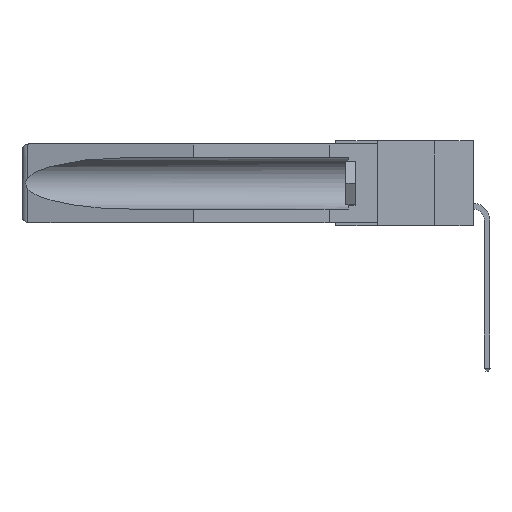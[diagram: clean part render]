
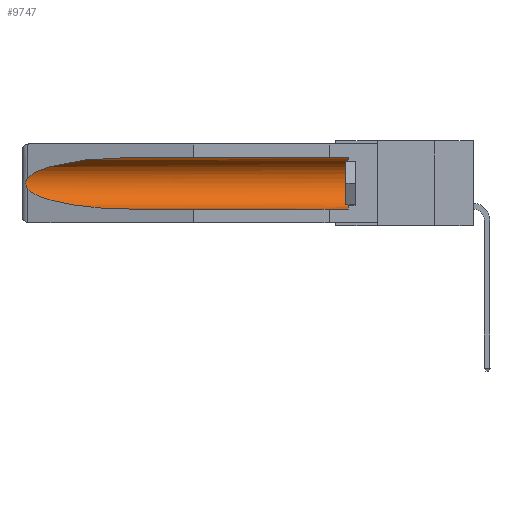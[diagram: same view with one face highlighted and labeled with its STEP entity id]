
A CAD part, left-side view. The second image highlights one B-rep face of the part: STEP entity #9747.
In plain terms, the highlighted cylindrical face has radius 2.857 mm (diameter 5.715 mm), a partial arc.
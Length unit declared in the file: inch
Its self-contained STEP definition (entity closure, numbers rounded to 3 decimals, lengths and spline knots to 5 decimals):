
#97 = CARTESIAN_POINT ( 'NONE',  ( 0.21114, 1.30732, -0.284 ) ) ;
#556 = CARTESIAN_POINT ( 'NONE',  ( 0.26537, 1.52718, -0.14972 ) ) ;
#1008 = DIRECTION ( 'NONE',  ( 0., -1., 0. ) ) ;
#1019 = CARTESIAN_POINT ( 'NONE',  ( 0.155, 0.126, -0.059 ) ) ;
#2188 = CARTESIAN_POINT ( 'NONE',  ( 0.155, 0.126, -0.284 ) ) ;
#2628 = CARTESIAN_POINT ( 'NONE',  ( 0.2673, 1.53269, -0.17917 ) ) ;
#2729 = CARTESIAN_POINT ( 'NONE',  ( 0.26537, 1.52718, -0.19328 ) ) ;
#3008 = FACE_OUTER_BOUND ( 'NONE', #10866, .T. ) ;
#3377 =( BOUNDED_CURVE ( )  B_SPLINE_CURVE ( 3, ( #17045, #12734, #97, #4221 ),
 .UNSPECIFIED., .F., .F. ) 
 B_SPLINE_CURVE_WITH_KNOTS ( ( 4, 4 ),
 ( 0.1948, 1.5708 ),
 .UNSPECIFIED. ) 
 CURVE ( )  GEOMETRIC_REPRESENTATION_ITEM ( )  RATIONAL_B_SPLINE_CURVE ( ( 1., 0.848, 0.848, 1. ) ) 
 REPRESENTATION_ITEM ( '' )  );
#3731 = VECTOR ( 'NONE', #23989, 39.37008 ) ;
#4221 = CARTESIAN_POINT ( 'NONE',  ( 0.155, 1.07973, -0.284 ) ) ;
#6785 = CARTESIAN_POINT ( 'NONE',  ( 0.26655, 1.53094, -0.18657 ) ) ;
#6896 = LINE ( 'NONE', #7996, #25304 ) ;
#7154 = CARTESIAN_POINT ( 'NONE',  ( 0.2675, 1.53308, -0.17534 ) ) ;
#7524 = CARTESIAN_POINT ( 'NONE',  ( 0.155, 1.07973, -0.059 ) ) ;
#7865 = CARTESIAN_POINT ( 'NONE',  ( 0.155, -0.30754, -0.1715 ) ) ;
#7996 = CARTESIAN_POINT ( 'NONE',  ( 0.155, -0.30754, -0.284 ) ) ;
#8344 =( BOUNDED_CURVE ( )  B_SPLINE_CURVE ( 3, ( #7524, #20384, #9386, #26865 ),
 .UNSPECIFIED., .F., .F. ) 
 B_SPLINE_CURVE_WITH_KNOTS ( ( 4, 4 ),
 ( 4.71239, 6.08839 ),
 .UNSPECIFIED. ) 
 CURVE ( )  GEOMETRIC_REPRESENTATION_ITEM ( )  RATIONAL_B_SPLINE_CURVE ( ( 1., 0.848, 0.848, 1. ) ) 
 REPRESENTATION_ITEM ( '' )  );
#8558 = DIRECTION ( 'NONE',  ( 0., 1., 0. ) ) ;
#8775 = AXIS2_PLACEMENT_3D ( 'NONE', #27025, #1008, #26660 ) ;
#8789 = VERTEX_POINT ( 'NONE', #556 ) ;
#8926 = CARTESIAN_POINT ( 'NONE',  ( 0.26654, 1.53092, -0.15636 ) ) ;
#9386 = CARTESIAN_POINT ( 'NONE',  ( 0.25451, 1.48313, -0.09465 ) ) ;
#9722 = ORIENTED_EDGE ( 'NONE', *, *, #15631, .T. ) ;
#9747 = ADVANCED_FACE ( 'NONE', ( #3008 ), #14406, .F. ) ;
#10416 = ORIENTED_EDGE ( 'NONE', *, *, #21142, .T. ) ;
#10866 = EDGE_LOOP ( 'NONE', ( #9722, #24416, #10416, #21864, #16224, #22308 ) ) ;
#11079 = CARTESIAN_POINT ( 'NONE',  ( 0.26597, 1.5296, -0.19026 ) ) ;
#11696 = EDGE_CURVE ( 'NONE', #16445, #13902, #19082, .T. ) ;
#12638 = CARTESIAN_POINT ( 'NONE',  ( 0.155, 1.07973, -0.284 ) ) ;
#12734 = CARTESIAN_POINT ( 'NONE',  ( 0.25451, 1.48313, -0.24835 ) ) ;
#13902 = VERTEX_POINT ( 'NONE', #1019 ) ;
#14406 = CYLINDRICAL_SURFACE ( 'NONE', #17858, 0.1125 ) ;
#15008 = CARTESIAN_POINT ( 'NONE',  ( 0.26537, 1.52718, -0.14972 ) ) ;
#15119 = VERTEX_POINT ( 'NONE', #19316 ) ;
#15456 = EDGE_CURVE ( 'NONE', #8789, #20237, #26883, .T. ) ;
#15473 = CARTESIAN_POINT ( 'NONE',  ( 0.2675, 1.53308, -0.16763 ) ) ;
#15631 = EDGE_CURVE ( 'NONE', #15119, #8789, #8344, .T. ) ;
#16224 = ORIENTED_EDGE ( 'NONE', *, *, #11696, .T. ) ;
#16445 = VERTEX_POINT ( 'NONE', #2188 ) ;
#16453 = DIRECTION ( 'NONE',  ( 0., 1., 0. ) ) ;
#17045 = CARTESIAN_POINT ( 'NONE',  ( 0.26537, 1.52718, -0.19328 ) ) ;
#17858 = AXIS2_PLACEMENT_3D ( 'NONE', #7865, #16453, #18582 ) ;
#18582 = DIRECTION ( 'NONE',  ( 0., 0., 1. ) ) ;
#18826 = EDGE_CURVE ( 'NONE', #13902, #15119, #20105, .T. ) ;
#19082 = CIRCLE ( 'NONE', #8775, 0.1125 ) ;
#19316 = CARTESIAN_POINT ( 'NONE',  ( 0.155, 1.07973, -0.059 ) ) ;
#19351 = VERTEX_POINT ( 'NONE', #12638 ) ;
#19736 = CARTESIAN_POINT ( 'NONE',  ( 0.26597, 1.52961, -0.15275 ) ) ;
#20105 = LINE ( 'NONE', #23539, #3731 ) ;
#20237 = VERTEX_POINT ( 'NONE', #26557 ) ;
#20384 = CARTESIAN_POINT ( 'NONE',  ( 0.21114, 1.30732, -0.059 ) ) ;
#21142 = EDGE_CURVE ( 'NONE', #20237, #19351, #3377, .T. ) ;
#21864 = ORIENTED_EDGE ( 'NONE', *, *, #22060, .F. ) ;
#21932 = CARTESIAN_POINT ( 'NONE',  ( 0.2673, 1.5327, -0.16383 ) ) ;
#22060 = EDGE_CURVE ( 'NONE', #16445, #19351, #6896, .T. ) ;
#22308 = ORIENTED_EDGE ( 'NONE', *, *, #18826, .T. ) ;
#23539 = CARTESIAN_POINT ( 'NONE',  ( 0.155, -0.30754, -0.059 ) ) ;
#23989 = DIRECTION ( 'NONE',  ( 0., 1., 0. ) ) ;
#24416 = ORIENTED_EDGE ( 'NONE', *, *, #15456, .T. ) ;
#25304 = VECTOR ( 'NONE', #8558, 39.37008 ) ;
#26557 = CARTESIAN_POINT ( 'NONE',  ( 0.26537, 1.52718, -0.19328 ) ) ;
#26660 = DIRECTION ( 'NONE',  ( 0., 0., 1. ) ) ;
#26865 = CARTESIAN_POINT ( 'NONE',  ( 0.26537, 1.52718, -0.14972 ) ) ;
#26883 = B_SPLINE_CURVE_WITH_KNOTS ( 'NONE', 3,
 ( #15008, #19736, #8926, #21932, #15473, #7154, #2628, #6785, #11079, #2729 ),
 .UNSPECIFIED., .F., .F.,
 ( 4, 2, 2, 2, 4 ),
 ( 0., 0.00029, 0.00058, 0.00087, 0.00117 ),
 .UNSPECIFIED. ) ;
#27025 = CARTESIAN_POINT ( 'NONE',  ( 0.155, 0.126, -0.1715 ) ) ;
